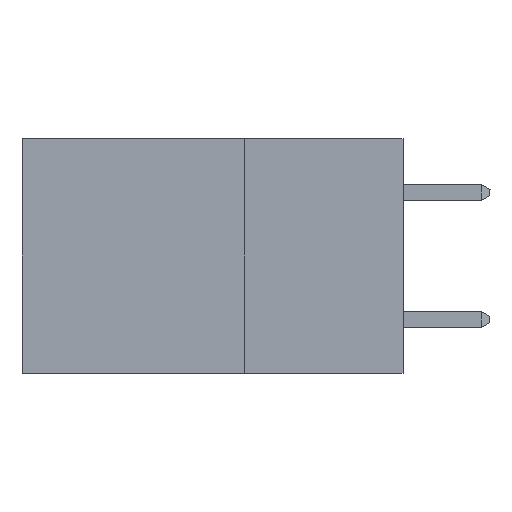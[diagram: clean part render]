
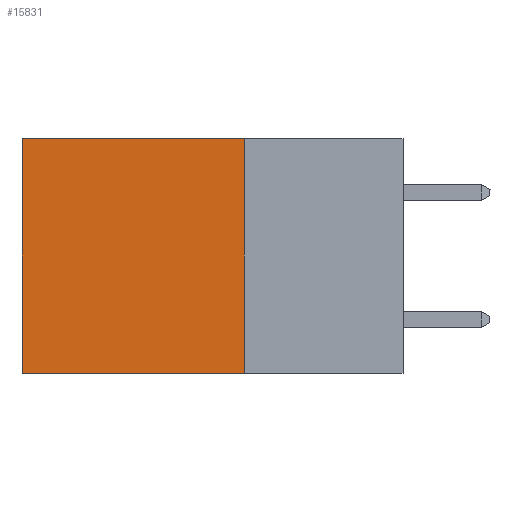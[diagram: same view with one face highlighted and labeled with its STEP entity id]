
A CAD part, left-side view. The second image highlights one B-rep face of the part: STEP entity #15831.
In plain terms, the highlighted planar face has unit normal (-1, 0, 0).
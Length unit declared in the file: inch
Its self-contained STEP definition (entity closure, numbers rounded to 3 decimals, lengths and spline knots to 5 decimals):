
#2588 = EDGE_CURVE ( 'NONE', #20458, #18895, #16908, .T. ) ;
#2673 = VECTOR ( 'NONE', #15434, 39.37008 ) ;
#4214 = CARTESIAN_POINT ( 'NONE',  ( 0.2875, 0.25, 0. ) ) ;
#4336 = DIRECTION ( 'NONE',  ( 1., 0., 0. ) ) ;
#4803 = CARTESIAN_POINT ( 'NONE',  ( 0.2875, 0.25, 0. ) ) ;
#6053 = VERTEX_POINT ( 'NONE', #22759 ) ;
#6833 = EDGE_CURVE ( 'NONE', #18463, #20458, #18855, .T. ) ;
#7248 = AXIS2_PLACEMENT_3D ( 'NONE', #4214, #4336, #19191 ) ;
#7834 = LINE ( 'NONE', #9874, #2673 ) ;
#9874 = CARTESIAN_POINT ( 'NONE',  ( 0.2875, 0.25, 0. ) ) ;
#10434 = LINE ( 'NONE', #16216, #21096 ) ;
#10553 = DIRECTION ( 'NONE',  ( 0., 1., 0. ) ) ;
#12723 = DIRECTION ( 'NONE',  ( 0., 1., 0. ) ) ;
#14218 = CARTESIAN_POINT ( 'NONE',  ( 0.2875, 0.6, 0. ) ) ;
#15404 = FACE_OUTER_BOUND ( 'NONE', #20868, .T. ) ;
#15434 = DIRECTION ( 'NONE',  ( 0., 0., -1. ) ) ;
#15490 = CARTESIAN_POINT ( 'NONE',  ( 0.2875, 0.6, -0.37 ) ) ;
#15831 = ADVANCED_FACE ( 'NONE', ( #15404 ), #22880, .F. ) ;
#16216 = CARTESIAN_POINT ( 'NONE',  ( 0.2875, 0.25, -0.37 ) ) ;
#16908 = LINE ( 'NONE', #22303, #17277 ) ;
#17145 = ORIENTED_EDGE ( 'NONE', *, *, #6833, .T. ) ;
#17277 = VECTOR ( 'NONE', #18257, 39.37008 ) ;
#17542 = ORIENTED_EDGE ( 'NONE', *, *, #21367, .F. ) ;
#18257 = DIRECTION ( 'NONE',  ( 0., 0., -1. ) ) ;
#18422 = ORIENTED_EDGE ( 'NONE', *, *, #2588, .T. ) ;
#18463 = VERTEX_POINT ( 'NONE', #4803 ) ;
#18855 = LINE ( 'NONE', #24306, #23458 ) ;
#18895 = VERTEX_POINT ( 'NONE', #15490 ) ;
#19191 = DIRECTION ( 'NONE',  ( 0., 0., -1. ) ) ;
#20066 = ORIENTED_EDGE ( 'NONE', *, *, #22126, .F. ) ;
#20458 = VERTEX_POINT ( 'NONE', #14218 ) ;
#20868 = EDGE_LOOP ( 'NONE', ( #18422, #17542, #20066, #17145 ) ) ;
#21096 = VECTOR ( 'NONE', #10553, 39.37008 ) ;
#21367 = EDGE_CURVE ( 'NONE', #6053, #18895, #10434, .T. ) ;
#22126 = EDGE_CURVE ( 'NONE', #18463, #6053, #7834, .T. ) ;
#22303 = CARTESIAN_POINT ( 'NONE',  ( 0.2875, 0.6, 0. ) ) ;
#22759 = CARTESIAN_POINT ( 'NONE',  ( 0.2875, 0.25, -0.37 ) ) ;
#22880 = PLANE ( 'NONE',  #7248 ) ;
#23458 = VECTOR ( 'NONE', #12723, 39.37008 ) ;
#24306 = CARTESIAN_POINT ( 'NONE',  ( 0.2875, 0.25, 0. ) ) ;
